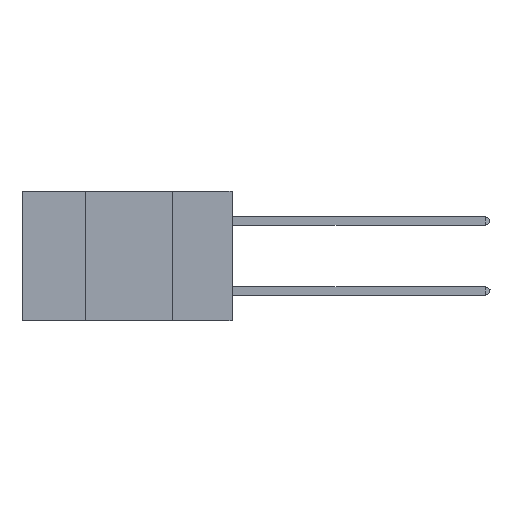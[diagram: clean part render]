
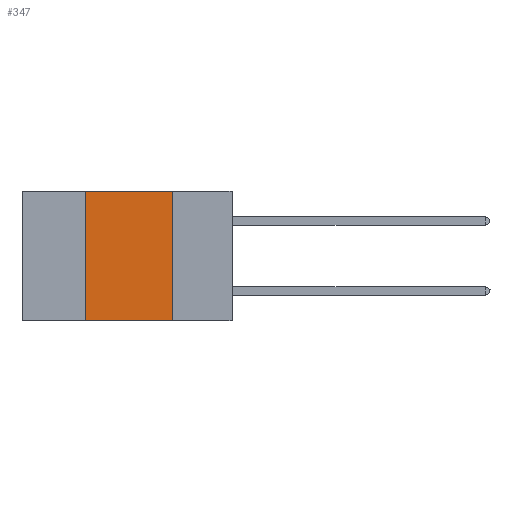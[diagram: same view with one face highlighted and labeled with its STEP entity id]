
A CAD part, left-side view. The second image highlights one B-rep face of the part: STEP entity #347.
In plain terms, the highlighted planar face has unit normal (-1, 0, 0).
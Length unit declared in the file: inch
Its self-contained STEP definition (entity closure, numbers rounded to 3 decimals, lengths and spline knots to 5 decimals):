
#194 = EDGE_CURVE ( 'NONE', #5666, #11224, #4762, .T. ) ;
#347 = ADVANCED_FACE ( 'NONE', ( #17496 ), #2363, .F. ) ;
#672 = ORIENTED_EDGE ( 'NONE', *, *, #10903, .F. ) ;
#744 = DIRECTION ( 'NONE',  ( 0., 0., -1. ) ) ;
#1308 = VECTOR ( 'NONE', #744, 39.37008 ) ;
#1792 = DIRECTION ( 'NONE',  ( 0., 0., 1. ) ) ;
#1999 = ORIENTED_EDGE ( 'NONE', *, *, #194, .F. ) ;
#2363 = PLANE ( 'NONE',  #8681 ) ;
#3463 = VECTOR ( 'NONE', #14120, 39.37008 ) ;
#4078 = EDGE_CURVE ( 'NONE', #17241, #6813, #4606, .T. ) ;
#4606 = LINE ( 'NONE', #4710, #3463 ) ;
#4710 = CARTESIAN_POINT ( 'NONE',  ( 0., 0.6, -0.37 ) ) ;
#4758 = LINE ( 'NONE', #17470, #15428 ) ;
#4762 = LINE ( 'NONE', #5038, #7115 ) ;
#5038 = CARTESIAN_POINT ( 'NONE',  ( 0., 0.6, 0. ) ) ;
#5649 = CARTESIAN_POINT ( 'NONE',  ( 0., 0.17, 0. ) ) ;
#5666 = VERTEX_POINT ( 'NONE', #8671 ) ;
#6326 = EDGE_LOOP ( 'NONE', ( #16662, #1999, #672, #16263 ) ) ;
#6787 = CARTESIAN_POINT ( 'NONE',  ( 0., 0.6, 0. ) ) ;
#6813 = VERTEX_POINT ( 'NONE', #12724 ) ;
#6925 = DIRECTION ( 'NONE',  ( 1., 0., 0. ) ) ;
#7115 = VECTOR ( 'NONE', #15393, 39.37008 ) ;
#8671 = CARTESIAN_POINT ( 'NONE',  ( 0., 0.42, 0. ) ) ;
#8681 = AXIS2_PLACEMENT_3D ( 'NONE', #6787, #6925, #14176 ) ;
#9615 = CARTESIAN_POINT ( 'NONE',  ( 0., 0.17, 0. ) ) ;
#10791 = CARTESIAN_POINT ( 'NONE',  ( 0., 0.42, -0.37 ) ) ;
#10903 = EDGE_CURVE ( 'NONE', #17241, #5666, #4758, .T. ) ;
#11224 = VERTEX_POINT ( 'NONE', #5649 ) ;
#12724 = CARTESIAN_POINT ( 'NONE',  ( 0., 0.17, -0.37 ) ) ;
#12883 = EDGE_CURVE ( 'NONE', #11224, #6813, #18672, .T. ) ;
#14120 = DIRECTION ( 'NONE',  ( 0., -1., 0. ) ) ;
#14176 = DIRECTION ( 'NONE',  ( 0., 0., -1. ) ) ;
#15393 = DIRECTION ( 'NONE',  ( 0., -1., 0. ) ) ;
#15428 = VECTOR ( 'NONE', #1792, 39.37008 ) ;
#16263 = ORIENTED_EDGE ( 'NONE', *, *, #4078, .T. ) ;
#16662 = ORIENTED_EDGE ( 'NONE', *, *, #12883, .F. ) ;
#17241 = VERTEX_POINT ( 'NONE', #10791 ) ;
#17470 = CARTESIAN_POINT ( 'NONE',  ( 0., 0.42, 0. ) ) ;
#17496 = FACE_OUTER_BOUND ( 'NONE', #6326, .T. ) ;
#18672 = LINE ( 'NONE', #9615, #1308 ) ;
